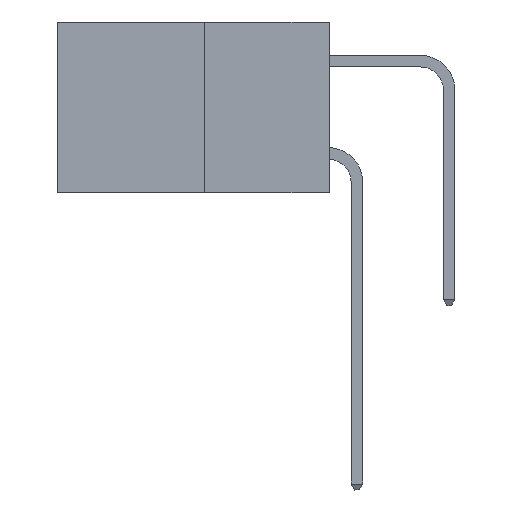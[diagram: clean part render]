
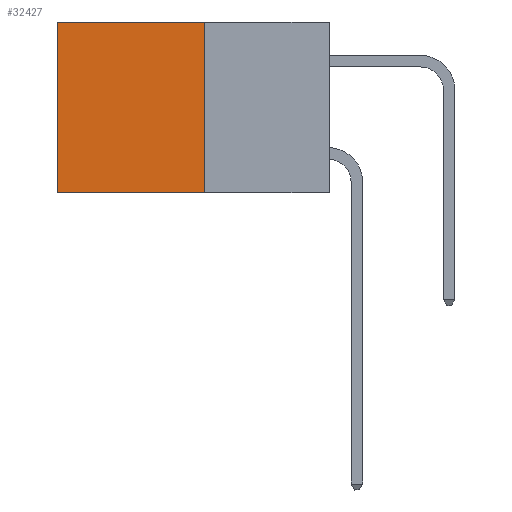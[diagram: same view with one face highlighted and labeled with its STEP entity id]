
A CAD part, left-side view. The second image highlights one B-rep face of the part: STEP entity #32427.
In plain terms, the highlighted planar face has unit normal (-1, 0, 0).
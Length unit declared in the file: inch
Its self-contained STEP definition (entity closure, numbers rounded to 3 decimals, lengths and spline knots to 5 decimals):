
#676 = CARTESIAN_POINT ( 'NONE',  ( 0.277, 0.27, 0. ) ) ;
#1490 = DIRECTION ( 'NONE',  ( 0., 1., 0. ) ) ;
#2656 = ORIENTED_EDGE ( 'NONE', *, *, #30531, .T. ) ;
#2918 = CARTESIAN_POINT ( 'NONE',  ( 0.277, 0.27, -0.37 ) ) ;
#3748 = DIRECTION ( 'NONE',  ( 0., 0., -1. ) ) ;
#4752 = VERTEX_POINT ( 'NONE', #22894 ) ;
#5601 = DIRECTION ( 'NONE',  ( 0., 0., -1. ) ) ;
#6437 = CARTESIAN_POINT ( 'NONE',  ( 0.277, 0.27, 0. ) ) ;
#7231 = FACE_OUTER_BOUND ( 'NONE', #27941, .T. ) ;
#9304 = VERTEX_POINT ( 'NONE', #23327 ) ;
#10577 = VECTOR ( 'NONE', #3748, 39.37008 ) ;
#12321 = ORIENTED_EDGE ( 'NONE', *, *, #15956, .F. ) ;
#12386 = VERTEX_POINT ( 'NONE', #19182 ) ;
#13528 = DIRECTION ( 'NONE',  ( 0., 0., -1. ) ) ;
#13589 = EDGE_CURVE ( 'NONE', #9304, #12386, #34375, .T. ) ;
#13921 = VECTOR ( 'NONE', #16739, 39.37008 ) ;
#15860 = EDGE_CURVE ( 'NONE', #15981, #4752, #28068, .T. ) ;
#15956 = EDGE_CURVE ( 'NONE', #15981, #9304, #19331, .T. ) ;
#15981 = VERTEX_POINT ( 'NONE', #6437 ) ;
#16739 = DIRECTION ( 'NONE',  ( 0., 1., 0. ) ) ;
#16999 = LINE ( 'NONE', #29443, #30260 ) ;
#19182 = CARTESIAN_POINT ( 'NONE',  ( 0.277, 0.59, -0.37 ) ) ;
#19331 = LINE ( 'NONE', #32946, #10577 ) ;
#20336 = VECTOR ( 'NONE', #1490, 39.37008 ) ;
#21590 = DIRECTION ( 'NONE',  ( 1., 0., 0. ) ) ;
#22481 = ORIENTED_EDGE ( 'NONE', *, *, #15860, .T. ) ;
#22894 = CARTESIAN_POINT ( 'NONE',  ( 0.277, 0.59, 0. ) ) ;
#23327 = CARTESIAN_POINT ( 'NONE',  ( 0.277, 0.27, -0.37 ) ) ;
#26280 = AXIS2_PLACEMENT_3D ( 'NONE', #2918, #21590, #5601 ) ;
#27941 = EDGE_LOOP ( 'NONE', ( #2656, #31214, #12321, #22481 ) ) ;
#28068 = LINE ( 'NONE', #676, #13921 ) ;
#29381 = PLANE ( 'NONE',  #26280 ) ;
#29443 = CARTESIAN_POINT ( 'NONE',  ( 0.277, 0.59, -0.37 ) ) ;
#30260 = VECTOR ( 'NONE', #13528, 39.37008 ) ;
#30531 = EDGE_CURVE ( 'NONE', #4752, #12386, #16999, .T. ) ;
#31214 = ORIENTED_EDGE ( 'NONE', *, *, #13589, .F. ) ;
#32427 = ADVANCED_FACE ( 'NONE', ( #7231 ), #29381, .F. ) ;
#32946 = CARTESIAN_POINT ( 'NONE',  ( 0.277, 0.27, -0.37 ) ) ;
#33389 = CARTESIAN_POINT ( 'NONE',  ( 0.277, 0.27, -0.37 ) ) ;
#34375 = LINE ( 'NONE', #33389, #20336 ) ;
